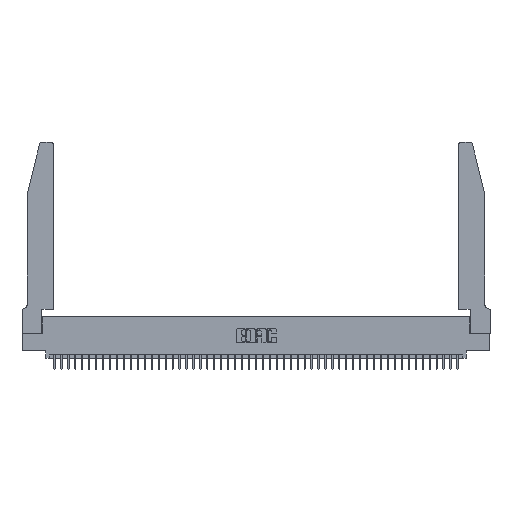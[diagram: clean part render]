
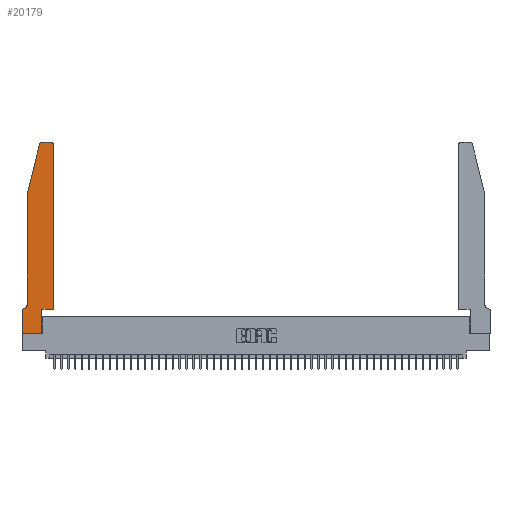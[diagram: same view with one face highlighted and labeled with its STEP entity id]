
A CAD part, top view. The second image highlights one B-rep face of the part: STEP entity #20179.
In plain terms, the highlighted planar face has unit normal (0, 0, 1).
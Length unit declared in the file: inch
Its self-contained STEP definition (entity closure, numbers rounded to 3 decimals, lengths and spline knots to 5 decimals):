
#442 = VERTEX_POINT ( 'NONE', #34289 ) ;
#733 = CARTESIAN_POINT ( 'NONE',  ( 0.0755, 2., 0.37 ) ) ;
#1046 = ORIENTED_EDGE ( 'NONE', *, *, #7974, .T. ) ;
#1451 = CARTESIAN_POINT ( 'NONE',  ( 0.4505, 2.72, 0.37 ) ) ;
#1547 = VERTEX_POINT ( 'NONE', #11623 ) ;
#1588 = CARTESIAN_POINT ( 'NONE',  ( 0.4505, 0.35, 0.37 ) ) ;
#1898 = DIRECTION ( 'NONE',  ( 0., 0., 1. ) ) ;
#2251 = CARTESIAN_POINT ( 'NONE',  ( 0.25487, 2.72718, 0.37 ) ) ;
#2276 = CARTESIAN_POINT ( 'NONE',  ( 0., 0., 0.37 ) ) ;
#2330 = LINE ( 'NONE', #17939, #17147 ) ;
#2390 = DIRECTION ( 'NONE',  ( 0., -1., 0. ) ) ;
#3159 = EDGE_CURVE ( 'NONE', #45158, #1547, #23174, .T. ) ;
#4154 = LINE ( 'NONE', #33421, #33175 ) ;
#4805 = CARTESIAN_POINT ( 'NONE',  ( 0.0055, 0.42, 0.37 ) ) ;
#5205 = EDGE_CURVE ( 'NONE', #32588, #37936, #20595, .T. ) ;
#5724 = DIRECTION ( 'NONE',  ( 1., 0., 0. ) ) ;
#7273 = CARTESIAN_POINT ( 'NONE',  ( 0.0755, 2., 0.37 ) ) ;
#7974 = EDGE_CURVE ( 'NONE', #12278, #35807, #39313, .T. ) ;
#8634 = CARTESIAN_POINT ( 'NONE',  ( 0.284, 2.75, 0.37 ) ) ;
#9029 = EDGE_LOOP ( 'NONE', ( #13812, #45921, #26123, #9172, #28975, #26957, #20072, #1046, #36250, #33788, #33343, #38901 ) ) ;
#9172 = ORIENTED_EDGE ( 'NONE', *, *, #3159, .T. ) ;
#9379 = CARTESIAN_POINT ( 'NONE',  ( 0., 0.35, 0.37 ) ) ;
#9713 = DIRECTION ( 'NONE',  ( -0.239, -0.971, 0. ) ) ;
#9738 = DIRECTION ( 'NONE',  ( 1., 0., 0. ) ) ;
#9888 = CARTESIAN_POINT ( 'NONE',  ( 0.0755, 2., 0.37 ) ) ;
#10693 = VECTOR ( 'NONE', #9713, 39.37008 ) ;
#11108 = DIRECTION ( 'NONE',  ( 0., 0., 1. ) ) ;
#11623 = CARTESIAN_POINT ( 'NONE',  ( 0.0755, 0.42, 0.37 ) ) ;
#11785 = CIRCLE ( 'NONE', #19203, 0.03 ) ;
#12278 = VERTEX_POINT ( 'NONE', #40084 ) ;
#12398 = DIRECTION ( 'NONE',  ( -1., 0., 0. ) ) ;
#13389 = LINE ( 'NONE', #17646, #32374 ) ;
#13617 = CARTESIAN_POINT ( 'NONE',  ( 0., 0., 0.37 ) ) ;
#13786 = CARTESIAN_POINT ( 'NONE',  ( 0.4205, 2.72, 0.37 ) ) ;
#13812 = ORIENTED_EDGE ( 'NONE', *, *, #47824, .T. ) ;
#15894 = EDGE_CURVE ( 'NONE', #1547, #32134, #21466, .T. ) ;
#17147 = VECTOR ( 'NONE', #36327, 39.37008 ) ;
#17359 = DIRECTION ( 'NONE',  ( 0., 1., 0. ) ) ;
#17622 = EDGE_CURVE ( 'NONE', #32134, #47222, #4154, .T. ) ;
#17646 = CARTESIAN_POINT ( 'NONE',  ( 0.4505, 0.35, 0.37 ) ) ;
#17939 = CARTESIAN_POINT ( 'NONE',  ( 0.2605, 2.75, 0.37 ) ) ;
#18087 = DIRECTION ( 'NONE',  ( 1., 0., 0. ) ) ;
#19203 = AXIS2_PLACEMENT_3D ( 'NONE', #13786, #1898, #5724 ) ;
#20072 = ORIENTED_EDGE ( 'NONE', *, *, #47928, .T. ) ;
#20179 = ADVANCED_FACE ( 'NONE', ( #24633 ), #22222, .T. ) ;
#20217 = DIRECTION ( 'NONE',  ( 0., 0., -1. ) ) ;
#20265 = CARTESIAN_POINT ( 'NONE',  ( 0.4505, 0.35, 0.37 ) ) ;
#20421 = DIRECTION ( 'NONE',  ( 0., 1., 0. ) ) ;
#20595 = CIRCLE ( 'NONE', #27675, 0.03 ) ;
#21354 = CARTESIAN_POINT ( 'NONE',  ( 0.284, 2.72, 0.37 ) ) ;
#21466 = CIRCLE ( 'NONE', #33154, 0.07 ) ;
#22222 = PLANE ( 'NONE',  #25012 ) ;
#23174 = LINE ( 'NONE', #7273, #42728 ) ;
#23812 = EDGE_CURVE ( 'NONE', #34942, #48974, #35692, .T. ) ;
#24633 = FACE_OUTER_BOUND ( 'NONE', #9029, .T. ) ;
#25012 = AXIS2_PLACEMENT_3D ( 'NONE', #40777, #11108, #18087 ) ;
#25917 = EDGE_CURVE ( 'NONE', #48974, #442, #11785, .T. ) ;
#26123 = ORIENTED_EDGE ( 'NONE', *, *, #34489, .T. ) ;
#26344 = DIRECTION ( 'NONE',  ( 0., -1., 0. ) ) ;
#26717 = CARTESIAN_POINT ( 'NONE',  ( 0.2865, 0., 0.37 ) ) ;
#26957 = ORIENTED_EDGE ( 'NONE', *, *, #17622, .T. ) ;
#27675 = AXIS2_PLACEMENT_3D ( 'NONE', #21354, #28811, #9738 ) ;
#27902 = LINE ( 'NONE', #9888, #10693 ) ;
#28261 = EDGE_CURVE ( 'NONE', #35807, #44604, #42947, .T. ) ;
#28811 = DIRECTION ( 'NONE',  ( 0., 0., 1. ) ) ;
#28912 = DIRECTION ( 'NONE',  ( 1., 0., 0. ) ) ;
#28975 = ORIENTED_EDGE ( 'NONE', *, *, #15894, .T. ) ;
#29621 = VECTOR ( 'NONE', #2390, 39.37008 ) ;
#30569 = EDGE_CURVE ( 'NONE', #44604, #34942, #13389, .T. ) ;
#32134 = VERTEX_POINT ( 'NONE', #43124 ) ;
#32374 = VECTOR ( 'NONE', #28912, 39.37008 ) ;
#32588 = VERTEX_POINT ( 'NONE', #8634 ) ;
#33154 = AXIS2_PLACEMENT_3D ( 'NONE', #4805, #20217, #12398 ) ;
#33175 = VECTOR ( 'NONE', #48253, 39.37008 ) ;
#33343 = ORIENTED_EDGE ( 'NONE', *, *, #23812, .T. ) ;
#33421 = CARTESIAN_POINT ( 'NONE',  ( 0.0755, 0.35, 0.37 ) ) ;
#33788 = ORIENTED_EDGE ( 'NONE', *, *, #30569, .T. ) ;
#34289 = CARTESIAN_POINT ( 'NONE',  ( 0.4205, 2.75, 0.37 ) ) ;
#34489 = EDGE_CURVE ( 'NONE', #37936, #45158, #27902, .T. ) ;
#34942 = VERTEX_POINT ( 'NONE', #1588 ) ;
#35227 = CARTESIAN_POINT ( 'NONE',  ( 0.2865, 0.35, 0.37 ) ) ;
#35692 = LINE ( 'NONE', #20265, #39255 ) ;
#35807 = VERTEX_POINT ( 'NONE', #26717 ) ;
#36108 = LINE ( 'NONE', #13617, #29621 ) ;
#36250 = ORIENTED_EDGE ( 'NONE', *, *, #28261, .T. ) ;
#36327 = DIRECTION ( 'NONE',  ( -1., 0., 0. ) ) ;
#36429 = VECTOR ( 'NONE', #17359, 39.37008 ) ;
#36868 = DIRECTION ( 'NONE',  ( 1., 0., 0. ) ) ;
#37575 = VECTOR ( 'NONE', #36868, 39.37008 ) ;
#37936 = VERTEX_POINT ( 'NONE', #2251 ) ;
#38901 = ORIENTED_EDGE ( 'NONE', *, *, #25917, .T. ) ;
#39255 = VECTOR ( 'NONE', #20421, 39.37008 ) ;
#39313 = LINE ( 'NONE', #2276, #37575 ) ;
#40084 = CARTESIAN_POINT ( 'NONE',  ( 0., 0., 0.37 ) ) ;
#40777 = CARTESIAN_POINT ( 'NONE',  ( 0., 0.35, 0.37 ) ) ;
#42728 = VECTOR ( 'NONE', #26344, 39.37008 ) ;
#42947 = LINE ( 'NONE', #43834, #36429 ) ;
#43124 = CARTESIAN_POINT ( 'NONE',  ( 0.0055, 0.35, 0.37 ) ) ;
#43834 = CARTESIAN_POINT ( 'NONE',  ( 0.2865, 0.35, 0.37 ) ) ;
#44604 = VERTEX_POINT ( 'NONE', #35227 ) ;
#45158 = VERTEX_POINT ( 'NONE', #733 ) ;
#45921 = ORIENTED_EDGE ( 'NONE', *, *, #5205, .T. ) ;
#47222 = VERTEX_POINT ( 'NONE', #9379 ) ;
#47824 = EDGE_CURVE ( 'NONE', #442, #32588, #2330, .T. ) ;
#47928 = EDGE_CURVE ( 'NONE', #47222, #12278, #36108, .T. ) ;
#48253 = DIRECTION ( 'NONE',  ( -1., 0., 0. ) ) ;
#48974 = VERTEX_POINT ( 'NONE', #1451 ) ;
